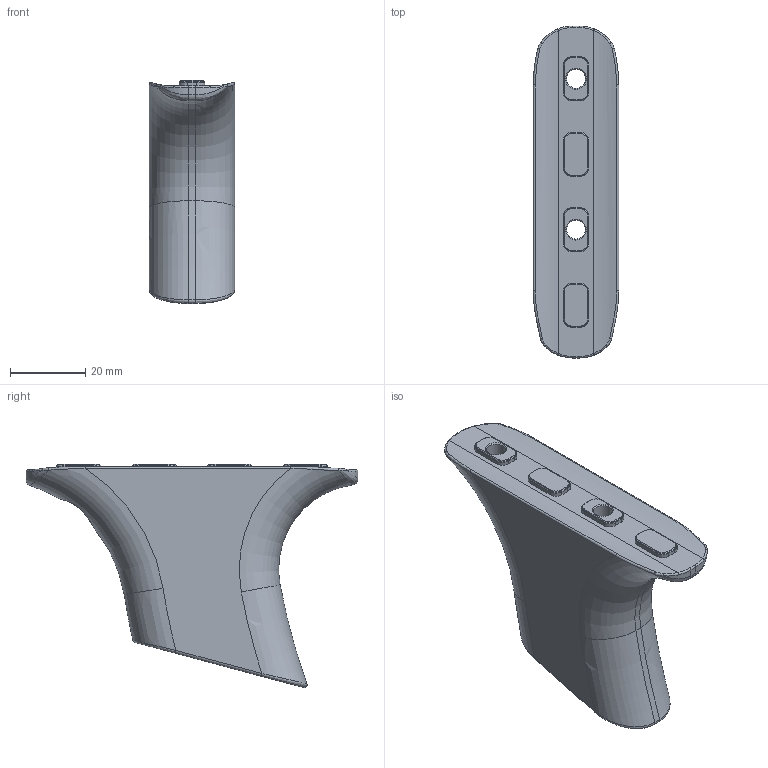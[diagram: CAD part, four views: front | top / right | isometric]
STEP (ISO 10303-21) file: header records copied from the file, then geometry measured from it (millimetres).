
FILE_DESCRIPTION(/* description */ (''),/* implementation_level */ '2;1');
FILE_NAME(/* name */ 'Standard.step',/* time_stamp */ '2021-10-28T08:45:54-04:00',/* author */ (''),/* organization */ (''),/* preprocessor_version */ 'ST-DEVELOPER v18.1',/* originating_system */ 'Autodesk Translation Framework v10.10.0.1391',/* authorisation */ '');
FILE_SCHEMA (('AUTOMOTIVE_DESIGN { 1 0 10303 214 3 1 1 }'));
Length unit declared in the file: millimetre
Products named in the file (1): Standard
Bounding box: 22.7 x 88 x 59.14 mm (x, y, z)
Volume: 35912.9 mm3; surface area: 14187.9 mm2
Topology: 1 solids, 1 shells, 258 faces, 584 edges, 338 vertices
Faces by surface type: cylinder 87, bspline 58, plane 57, torus 38, cone 18
Full cylindrical faces by diameter (mm): 5 x2, 9.3 x2, 12.778 x1, 14.758 x1
Entity records: 9166 total; most frequent: CARTESIAN_POINT 3575, ORIENTED_EDGE 1168, DIRECTION 1136, EDGE_CURVE 584, AXIS2_PLACEMENT_3D 459, VERTEX_POINT 338, EDGE_LOOP 272, FACE_OUTER_BOUND 258
